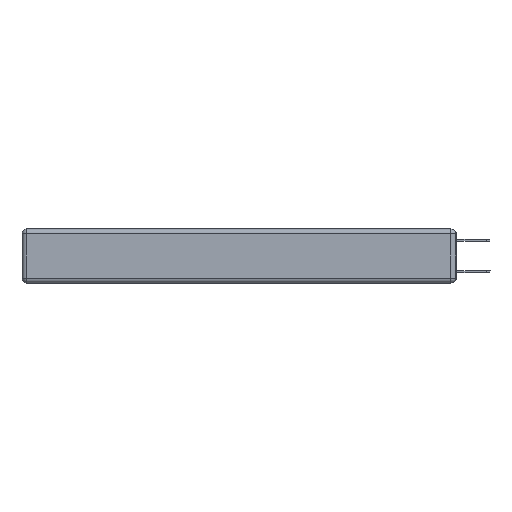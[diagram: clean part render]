
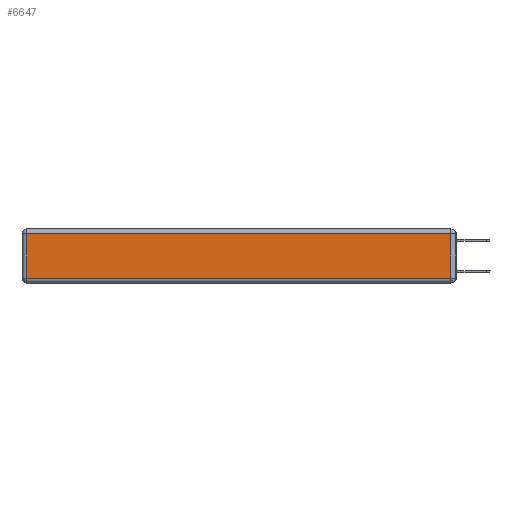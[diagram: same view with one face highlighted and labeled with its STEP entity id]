
A CAD part, left-side view. The second image highlights one B-rep face of the part: STEP entity #6647.
In plain terms, the highlighted planar face has unit normal (-1, 0, 0).
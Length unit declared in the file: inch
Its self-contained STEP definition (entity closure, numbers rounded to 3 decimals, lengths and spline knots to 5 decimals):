
#175 = EDGE_LOOP ( 'NONE', ( #8926, #8676, #358, #8524 ) ) ;
#358 = ORIENTED_EDGE ( 'NONE', *, *, #5526, .T. ) ;
#1025 = AXIS2_PLACEMENT_3D ( 'NONE', #6774, #6814, #12175 ) ;
#1058 = CARTESIAN_POINT ( 'NONE',  ( 0., 0., -0.313 ) ) ;
#2112 = VERTEX_POINT ( 'NONE', #7702 ) ;
#2144 = VECTOR ( 'NONE', #3930, 39.37008 ) ;
#2505 = DIRECTION ( 'NONE',  ( 0., 1., 0. ) ) ;
#2580 = EDGE_CURVE ( 'NONE', #5842, #2112, #11492, .T. ) ;
#2982 = VERTEX_POINT ( 'NONE', #9077 ) ;
#3288 = CARTESIAN_POINT ( 'NONE',  ( 0., 0.03, -0.03 ) ) ;
#3596 = CARTESIAN_POINT ( 'NONE',  ( 0., 2.72, -0.343 ) ) ;
#3890 = CARTESIAN_POINT ( 'NONE',  ( 0., 0.03, -0.343 ) ) ;
#3930 = DIRECTION ( 'NONE',  ( 0., 0., 1. ) ) ;
#4022 = CARTESIAN_POINT ( 'NONE',  ( 0., 2.72, -0.313 ) ) ;
#4345 = LINE ( 'NONE', #3890, #2144 ) ;
#4361 = FACE_OUTER_BOUND ( 'NONE', #175, .T. ) ;
#4505 = VECTOR ( 'NONE', #6580, 39.37008 ) ;
#4686 = PLANE ( 'NONE',  #1025 ) ;
#5022 = DIRECTION ( 'NONE',  ( 0., 0., -1. ) ) ;
#5526 = EDGE_CURVE ( 'NONE', #9928, #2982, #10041, .T. ) ;
#5842 = VERTEX_POINT ( 'NONE', #4022 ) ;
#6580 = DIRECTION ( 'NONE',  ( 0., -1., 0. ) ) ;
#6647 = ADVANCED_FACE ( 'NONE', ( #4361 ), #4686, .T. ) ;
#6774 = CARTESIAN_POINT ( 'NONE',  ( 0., 0., -0.343 ) ) ;
#6794 = VECTOR ( 'NONE', #2505, 39.37008 ) ;
#6814 = DIRECTION ( 'NONE',  ( -1., 0., 0. ) ) ;
#6976 = EDGE_CURVE ( 'NONE', #2112, #9928, #4345, .T. ) ;
#7702 = CARTESIAN_POINT ( 'NONE',  ( 0., 0.03, -0.313 ) ) ;
#8524 = ORIENTED_EDGE ( 'NONE', *, *, #13614, .T. ) ;
#8676 = ORIENTED_EDGE ( 'NONE', *, *, #6976, .T. ) ;
#8839 = VECTOR ( 'NONE', #5022, 39.37008 ) ;
#8926 = ORIENTED_EDGE ( 'NONE', *, *, #2580, .T. ) ;
#9077 = CARTESIAN_POINT ( 'NONE',  ( 0., 2.72, -0.03 ) ) ;
#9138 = LINE ( 'NONE', #3596, #8839 ) ;
#9928 = VERTEX_POINT ( 'NONE', #3288 ) ;
#10041 = LINE ( 'NONE', #12173, #6794 ) ;
#11492 = LINE ( 'NONE', #1058, #4505 ) ;
#12173 = CARTESIAN_POINT ( 'NONE',  ( 0., 2.75, -0.03 ) ) ;
#12175 = DIRECTION ( 'NONE',  ( 0., 0., 1. ) ) ;
#13614 = EDGE_CURVE ( 'NONE', #2982, #5842, #9138, .T. ) ;
